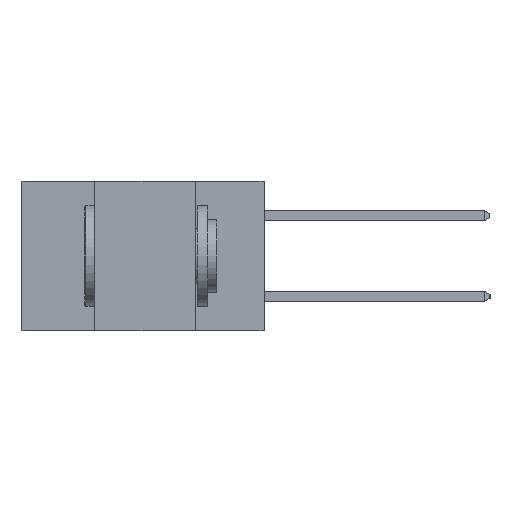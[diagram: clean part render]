
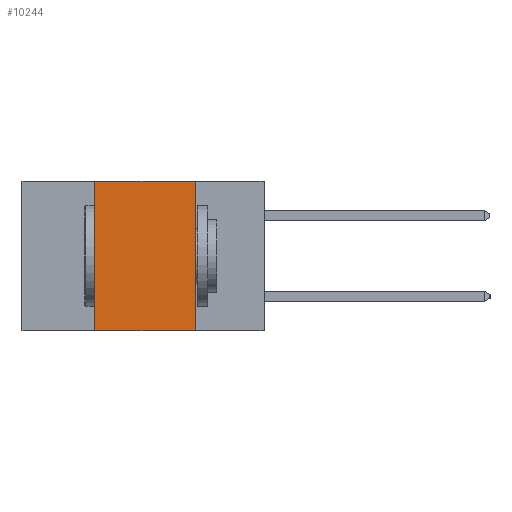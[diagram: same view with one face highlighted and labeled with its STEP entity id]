
A CAD part, left-side view. The second image highlights one B-rep face of the part: STEP entity #10244.
In plain terms, the highlighted planar face has unit normal (-1, 0, 0).
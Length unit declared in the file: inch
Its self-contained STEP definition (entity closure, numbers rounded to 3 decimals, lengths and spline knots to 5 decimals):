
#1104 = DIRECTION ( 'NONE',  ( 1., 0., 0. ) ) ;
#1573 = DIRECTION ( 'NONE',  ( 0., 0., -1. ) ) ;
#1741 = CARTESIAN_POINT ( 'NONE',  ( 0., 0.17, 0. ) ) ;
#2666 = EDGE_LOOP ( 'NONE', ( #22434, #3058, #16483, #9708 ) ) ;
#3058 = ORIENTED_EDGE ( 'NONE', *, *, #8125, .F. ) ;
#4035 = LINE ( 'NONE', #10087, #8827 ) ;
#4244 = DIRECTION ( 'NONE',  ( 0., -1., 0. ) ) ;
#4266 = CARTESIAN_POINT ( 'NONE',  ( 0., 0.6, 0. ) ) ;
#5704 = EDGE_CURVE ( 'NONE', #9903, #17552, #9945, .T. ) ;
#8125 = EDGE_CURVE ( 'NONE', #12603, #14493, #15104, .T. ) ;
#8199 = CARTESIAN_POINT ( 'NONE',  ( 0., 0.42, -0.37 ) ) ;
#8396 = VECTOR ( 'NONE', #4244, 39.37008 ) ;
#8827 = VECTOR ( 'NONE', #26230, 39.37008 ) ;
#9315 = VECTOR ( 'NONE', #12727, 39.37008 ) ;
#9708 = ORIENTED_EDGE ( 'NONE', *, *, #5704, .T. ) ;
#9903 = VERTEX_POINT ( 'NONE', #8199 ) ;
#9945 = LINE ( 'NONE', #12983, #9315 ) ;
#10087 = CARTESIAN_POINT ( 'NONE',  ( 0., 0.42, -0.37 ) ) ;
#10244 = ADVANCED_FACE ( 'NONE', ( #12166 ), #21403, .F. ) ;
#12166 = FACE_OUTER_BOUND ( 'NONE', #2666, .T. ) ;
#12405 = VECTOR ( 'NONE', #1573, 39.37008 ) ;
#12603 = VERTEX_POINT ( 'NONE', #16566 ) ;
#12727 = DIRECTION ( 'NONE',  ( 0., -1., 0. ) ) ;
#12983 = CARTESIAN_POINT ( 'NONE',  ( 0., 0.6, -0.37 ) ) ;
#13389 = CARTESIAN_POINT ( 'NONE',  ( 0., 0.6, 0. ) ) ;
#14440 = EDGE_CURVE ( 'NONE', #14493, #17552, #23744, .T. ) ;
#14493 = VERTEX_POINT ( 'NONE', #1741 ) ;
#14981 = CARTESIAN_POINT ( 'NONE',  ( 0., 0.17, -0.37 ) ) ;
#15104 = LINE ( 'NONE', #4266, #8396 ) ;
#15293 = EDGE_CURVE ( 'NONE', #9903, #12603, #4035, .T. ) ;
#15407 = DIRECTION ( 'NONE',  ( 0., 0., -1. ) ) ;
#15783 = CARTESIAN_POINT ( 'NONE',  ( 0., 0.17, -0.37 ) ) ;
#16483 = ORIENTED_EDGE ( 'NONE', *, *, #15293, .F. ) ;
#16566 = CARTESIAN_POINT ( 'NONE',  ( 0., 0.42, 0. ) ) ;
#17552 = VERTEX_POINT ( 'NONE', #14981 ) ;
#20870 = AXIS2_PLACEMENT_3D ( 'NONE', #13389, #1104, #15407 ) ;
#21403 = PLANE ( 'NONE',  #20870 ) ;
#22434 = ORIENTED_EDGE ( 'NONE', *, *, #14440, .F. ) ;
#23744 = LINE ( 'NONE', #15783, #12405 ) ;
#26230 = DIRECTION ( 'NONE',  ( 0., 0., 1. ) ) ;
